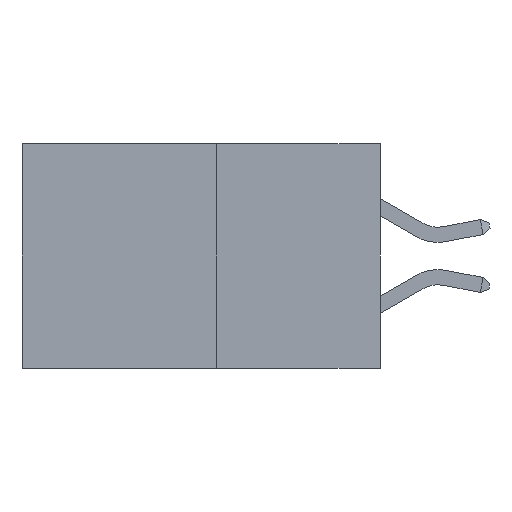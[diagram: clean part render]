
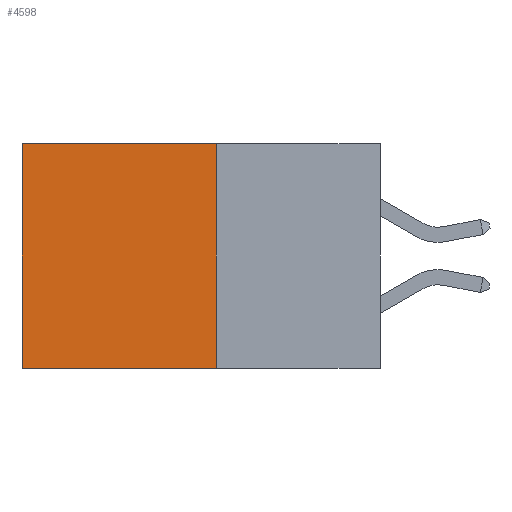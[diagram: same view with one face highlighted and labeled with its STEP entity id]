
A CAD part, left-side view. The second image highlights one B-rep face of the part: STEP entity #4598.
In plain terms, the highlighted planar face has unit normal (-1, 0, 0).
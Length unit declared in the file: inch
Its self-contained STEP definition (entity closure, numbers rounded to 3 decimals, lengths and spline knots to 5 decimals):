
#62 = CARTESIAN_POINT ( 'NONE',  ( 0.277, 0.27, 0. ) ) ;
#219 = VECTOR ( 'NONE', #2541, 39.37008 ) ;
#644 = VECTOR ( 'NONE', #6426, 39.37008 ) ;
#978 = VERTEX_POINT ( 'NONE', #4344 ) ;
#1410 = LINE ( 'NONE', #1574, #7825 ) ;
#1574 = CARTESIAN_POINT ( 'NONE',  ( 0.277, 0.27, -0.37 ) ) ;
#2255 = EDGE_CURVE ( 'NONE', #4588, #2964, #3765, .T. ) ;
#2344 = LINE ( 'NONE', #4534, #3854 ) ;
#2440 = ORIENTED_EDGE ( 'NONE', *, *, #2563, .F. ) ;
#2497 = EDGE_LOOP ( 'NONE', ( #4213, #2440, #3999, #3256 ) ) ;
#2541 = DIRECTION ( 'NONE',  ( 0., 0., -1. ) ) ;
#2563 = EDGE_CURVE ( 'NONE', #978, #2964, #7244, .T. ) ;
#2634 = EDGE_CURVE ( 'NONE', #3435, #978, #1410, .T. ) ;
#2751 = EDGE_CURVE ( 'NONE', #3435, #4588, #2344, .T. ) ;
#2918 = CARTESIAN_POINT ( 'NONE',  ( 0.277, 0.59, 0. ) ) ;
#2964 = VERTEX_POINT ( 'NONE', #7242 ) ;
#3256 = ORIENTED_EDGE ( 'NONE', *, *, #2751, .T. ) ;
#3308 = CARTESIAN_POINT ( 'NONE',  ( 0.277, 0.59, -0.37 ) ) ;
#3435 = VERTEX_POINT ( 'NONE', #62 ) ;
#3765 = LINE ( 'NONE', #3308, #219 ) ;
#3854 = VECTOR ( 'NONE', #5659, 39.37008 ) ;
#3999 = ORIENTED_EDGE ( 'NONE', *, *, #2634, .F. ) ;
#4213 = ORIENTED_EDGE ( 'NONE', *, *, #2255, .T. ) ;
#4344 = CARTESIAN_POINT ( 'NONE',  ( 0.277, 0.27, -0.37 ) ) ;
#4534 = CARTESIAN_POINT ( 'NONE',  ( 0.277, 0.27, 0. ) ) ;
#4588 = VERTEX_POINT ( 'NONE', #2918 ) ;
#4598 = ADVANCED_FACE ( 'NONE', ( #7809 ), #7799, .F. ) ;
#4732 = AXIS2_PLACEMENT_3D ( 'NONE', #7481, #7463, #5589 ) ;
#5589 = DIRECTION ( 'NONE',  ( 0., 0., -1. ) ) ;
#5659 = DIRECTION ( 'NONE',  ( 0., 1., 0. ) ) ;
#6180 = CARTESIAN_POINT ( 'NONE',  ( 0.277, 0.27, -0.37 ) ) ;
#6426 = DIRECTION ( 'NONE',  ( 0., 1., 0. ) ) ;
#7242 = CARTESIAN_POINT ( 'NONE',  ( 0.277, 0.59, -0.37 ) ) ;
#7244 = LINE ( 'NONE', #6180, #644 ) ;
#7298 = DIRECTION ( 'NONE',  ( 0., 0., -1. ) ) ;
#7463 = DIRECTION ( 'NONE',  ( 1., 0., 0. ) ) ;
#7481 = CARTESIAN_POINT ( 'NONE',  ( 0.277, 0.27, -0.37 ) ) ;
#7799 = PLANE ( 'NONE',  #4732 ) ;
#7809 = FACE_OUTER_BOUND ( 'NONE', #2497, .T. ) ;
#7825 = VECTOR ( 'NONE', #7298, 39.37008 ) ;
